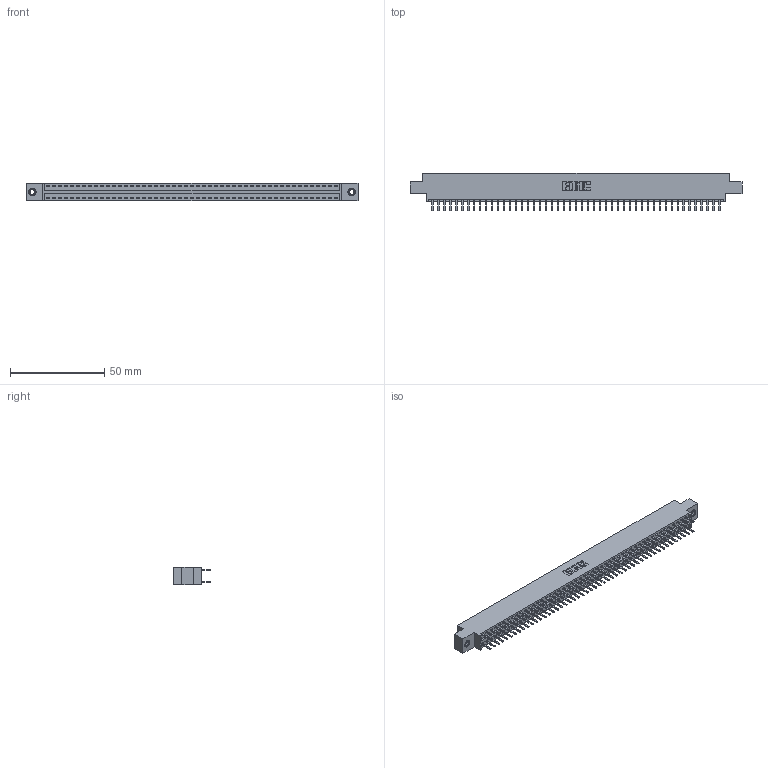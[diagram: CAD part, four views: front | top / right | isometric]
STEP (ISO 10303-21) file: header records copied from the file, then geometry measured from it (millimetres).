
FILE_DESCRIPTION (( 'STEP AP203' ), '1' );
FILE_NAME ('396-098-520-807.STEP', '2018-09-14T04:15:06', ( '' ), ( '' ), 'SwSTEP 2.0', 'SolidWorks 2016', '' );
FILE_SCHEMA (( 'CONFIG_CONTROL_DESIGN' ));
Length unit declared in the file: inch
Products named in the file (4): 346 Part_0.170 Offset - 0.156 Dia-TI; 345-292-001_345-293-120; 345-250-001_345-250-005-103; 396-098-520-807
Assembly tree (101 placements, depth 2):
  396-098-520-807
    346 Part_0.170 Offset - 0.156 Dia-TI
    345-292-001_345-293-120  x98
    345-250-001_345-250-005-103  x2
Bounding box: 176.15 x 20.02 x 9.4 mm (x, y, z)
Volume: 17019.9 mm3; surface area: 23617.4 mm2
Topology: 101 solids, 101 shells, 5674 faces, 16451 edges, 10698 vertices
Faces by surface type: plane 3738, cylinder 1920, cone 12, torus 4
Entity records: 32468 total; most frequent: CARTESIAN_POINT 5339, ORIENTED_EDGE 5254, DIRECTION 4769, EDGE_CURVE 2627, VECTOR 2275, LINE 2275, VERTEX_POINT 1744, AXIS2_PLACEMENT_3D 1247
